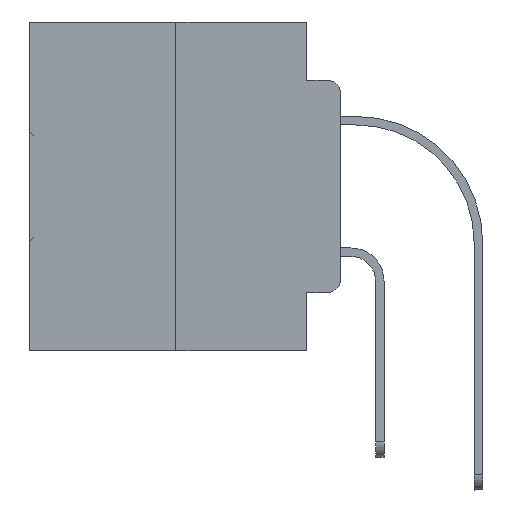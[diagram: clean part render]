
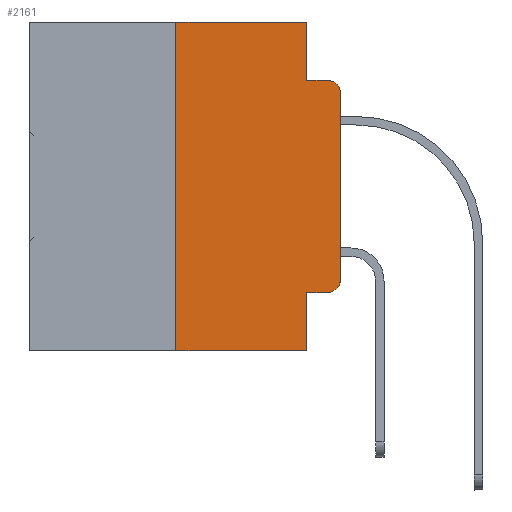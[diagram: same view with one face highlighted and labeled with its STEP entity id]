
A CAD part, left-side view. The second image highlights one B-rep face of the part: STEP entity #2161.
In plain terms, the highlighted planar face has unit normal (-1, 0, 0).
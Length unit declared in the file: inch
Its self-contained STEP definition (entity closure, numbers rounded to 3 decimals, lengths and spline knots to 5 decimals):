
#997 = VERTEX_POINT ( 'NONE', #28713 ) ;
#2148 = ORIENTED_EDGE ( 'NONE', *, *, #21851, .F. ) ;
#2161 = ADVANCED_FACE ( 'NONE', ( #5759 ), #19697, .F. ) ;
#2214 = CARTESIAN_POINT ( 'NONE',  ( 0., 0., 0. ) ) ;
#2561 = ORIENTED_EDGE ( 'NONE', *, *, #32747, .T. ) ;
#2681 = VERTEX_POINT ( 'NONE', #5552 ) ;
#3183 = CARTESIAN_POINT ( 'NONE',  ( 0., 0.473, -0.5 ) ) ;
#3441 = EDGE_CURVE ( 'NONE', #19769, #21257, #35600, .T. ) ;
#3704 = LINE ( 'NONE', #12178, #16417 ) ;
#4171 = CARTESIAN_POINT ( 'NONE',  ( 0., 0.25, 0. ) ) ;
#4519 = VERTEX_POINT ( 'NONE', #8993 ) ;
#4916 = CARTESIAN_POINT ( 'NONE',  ( 0., 0.25, 0. ) ) ;
#4992 = DIRECTION ( 'NONE',  ( 0., 0., -1. ) ) ;
#5024 = CARTESIAN_POINT ( 'NONE',  ( 0., 0.02, -0.3915 ) ) ;
#5107 = EDGE_CURVE ( 'NONE', #9755, #19769, #3704, .T. ) ;
#5136 = EDGE_LOOP ( 'NONE', ( #30352, #27477, #27124, #29247, #7242, #2148, #31679, #5368, #34189, #2561 ) ) ;
#5368 = ORIENTED_EDGE ( 'NONE', *, *, #10213, .F. ) ;
#5552 = CARTESIAN_POINT ( 'NONE',  ( 0., 0.02, -0.4115 ) ) ;
#5759 = FACE_OUTER_BOUND ( 'NONE', #5136, .T. ) ;
#6715 = AXIS2_PLACEMENT_3D ( 'NONE', #10805, #15528, #32585 ) ;
#7237 = LINE ( 'NONE', #4171, #10587 ) ;
#7242 = ORIENTED_EDGE ( 'NONE', *, *, #22964, .F. ) ;
#8617 = VECTOR ( 'NONE', #4992, 39.37008 ) ;
#8993 = CARTESIAN_POINT ( 'NONE',  ( 0., 0., -0.1085 ) ) ;
#9634 = DIRECTION ( 'NONE',  ( 0., -1., 0. ) ) ;
#9755 = VERTEX_POINT ( 'NONE', #26969 ) ;
#10079 = DIRECTION ( 'NONE',  ( 0., 0., -1. ) ) ;
#10213 = EDGE_CURVE ( 'NONE', #28251, #997, #18558, .T. ) ;
#10235 = CARTESIAN_POINT ( 'NONE',  ( 0., 0.051, -0.0885 ) ) ;
#10587 = VECTOR ( 'NONE', #15744, 39.37008 ) ;
#10805 = CARTESIAN_POINT ( 'NONE',  ( 0., 0.02, -0.1085 ) ) ;
#11357 = CARTESIAN_POINT ( 'NONE',  ( 0., 0.473, 0. ) ) ;
#11672 = VECTOR ( 'NONE', #18997, 39.37008 ) ;
#11997 = DIRECTION ( 'NONE',  ( 0., 0., -1. ) ) ;
#12178 = CARTESIAN_POINT ( 'NONE',  ( 0., 0.051, 0. ) ) ;
#12343 = LINE ( 'NONE', #23417, #22798 ) ;
#12645 = EDGE_CURVE ( 'NONE', #35639, #4519, #35685, .T. ) ;
#13119 = CARTESIAN_POINT ( 'NONE',  ( 0., 0.051, 0. ) ) ;
#14604 = DIRECTION ( 'NONE',  ( 1., 0., 0. ) ) ;
#15528 = DIRECTION ( 'NONE',  ( -1., 0., 0. ) ) ;
#15744 = DIRECTION ( 'NONE',  ( 0., 0., 1. ) ) ;
#16417 = VECTOR ( 'NONE', #11997, 39.37008 ) ;
#16629 = CARTESIAN_POINT ( 'NONE',  ( 0., 0.051, -0.4115 ) ) ;
#16701 = CARTESIAN_POINT ( 'NONE',  ( 0., 0.02, -0.0885 ) ) ;
#17162 = AXIS2_PLACEMENT_3D ( 'NONE', #11357, #14604, #28057 ) ;
#18558 = LINE ( 'NONE', #13119, #8617 ) ;
#18997 = DIRECTION ( 'NONE',  ( 0., -1., 0. ) ) ;
#19600 = CARTESIAN_POINT ( 'NONE',  ( 0., 0.051, -0.0885 ) ) ;
#19697 = PLANE ( 'NONE',  #17162 ) ;
#19769 = VERTEX_POINT ( 'NONE', #19600 ) ;
#20779 = DIRECTION ( 'NONE',  ( -1., 0., 0. ) ) ;
#21257 = VERTEX_POINT ( 'NONE', #16701 ) ;
#21675 = LINE ( 'NONE', #3183, #31298 ) ;
#21838 = DIRECTION ( 'NONE',  ( 0., -1., 0. ) ) ;
#21851 = EDGE_CURVE ( 'NONE', #30696, #27517, #7237, .T. ) ;
#22798 = VECTOR ( 'NONE', #9634, 39.37008 ) ;
#22964 = EDGE_CURVE ( 'NONE', #27517, #9755, #12343, .T. ) ;
#23250 = CARTESIAN_POINT ( 'NONE',  ( 0., 0.051, -0.4115 ) ) ;
#23417 = CARTESIAN_POINT ( 'NONE',  ( 0., 0.473, 0. ) ) ;
#25150 = CARTESIAN_POINT ( 'NONE',  ( 0., 0.25, -0.5 ) ) ;
#26648 = EDGE_CURVE ( 'NONE', #4519, #21257, #31603, .T. ) ;
#26924 = VECTOR ( 'NONE', #21838, 39.37008 ) ;
#26969 = CARTESIAN_POINT ( 'NONE',  ( 0., 0.051, 0. ) ) ;
#27124 = ORIENTED_EDGE ( 'NONE', *, *, #3441, .F. ) ;
#27207 = DIRECTION ( 'NONE',  ( 0., 0., 1. ) ) ;
#27477 = ORIENTED_EDGE ( 'NONE', *, *, #26648, .T. ) ;
#27517 = VERTEX_POINT ( 'NONE', #4916 ) ;
#27717 = LINE ( 'NONE', #16629, #11672 ) ;
#27838 = DIRECTION ( 'NONE',  ( 0., -1., 0. ) ) ;
#28057 = DIRECTION ( 'NONE',  ( 0., 0., -1. ) ) ;
#28251 = VERTEX_POINT ( 'NONE', #23250 ) ;
#28477 = CIRCLE ( 'NONE', #31947, 0.02 ) ;
#28713 = CARTESIAN_POINT ( 'NONE',  ( 0., 0.051, -0.5 ) ) ;
#29247 = ORIENTED_EDGE ( 'NONE', *, *, #5107, .F. ) ;
#30352 = ORIENTED_EDGE ( 'NONE', *, *, #12645, .T. ) ;
#30696 = VERTEX_POINT ( 'NONE', #25150 ) ;
#31165 = EDGE_CURVE ( 'NONE', #30696, #997, #21675, .T. ) ;
#31298 = VECTOR ( 'NONE', #27838, 39.37008 ) ;
#31344 = VECTOR ( 'NONE', #27207, 39.37008 ) ;
#31603 = CIRCLE ( 'NONE', #6715, 0.02 ) ;
#31679 = ORIENTED_EDGE ( 'NONE', *, *, #31165, .T. ) ;
#31947 = AXIS2_PLACEMENT_3D ( 'NONE', #5024, #20779, #10079 ) ;
#32585 = DIRECTION ( 'NONE',  ( 0., 0., -1. ) ) ;
#32747 = EDGE_CURVE ( 'NONE', #2681, #35639, #28477, .T. ) ;
#34189 = ORIENTED_EDGE ( 'NONE', *, *, #35615, .T. ) ;
#35600 = LINE ( 'NONE', #10235, #26924 ) ;
#35615 = EDGE_CURVE ( 'NONE', #28251, #2681, #27717, .T. ) ;
#35639 = VERTEX_POINT ( 'NONE', #35667 ) ;
#35667 = CARTESIAN_POINT ( 'NONE',  ( 0., 0., -0.3915 ) ) ;
#35685 = LINE ( 'NONE', #2214, #31344 ) ;
